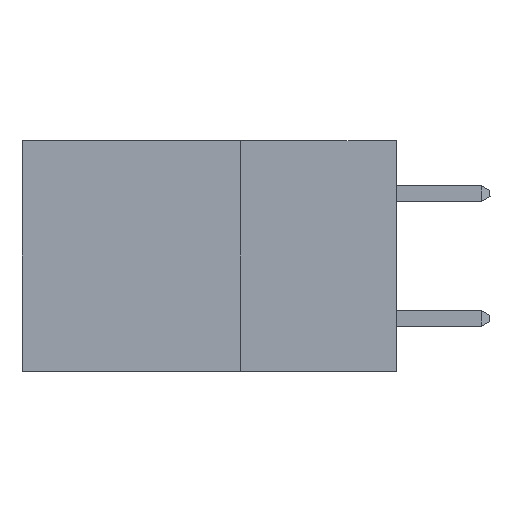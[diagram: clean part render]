
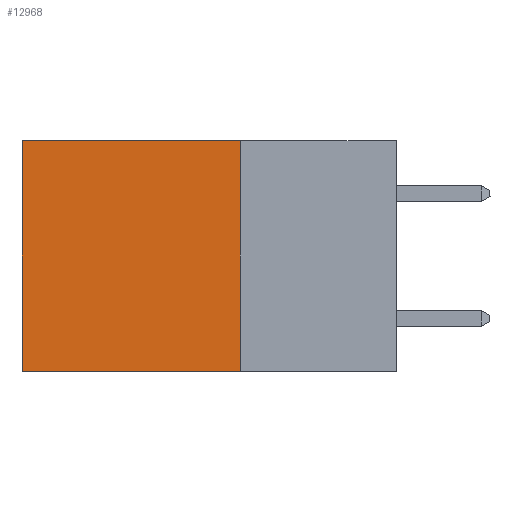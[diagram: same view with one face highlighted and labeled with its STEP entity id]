
A CAD part, left-side view. The second image highlights one B-rep face of the part: STEP entity #12968.
In plain terms, the highlighted planar face has unit normal (-1, 0, 0).
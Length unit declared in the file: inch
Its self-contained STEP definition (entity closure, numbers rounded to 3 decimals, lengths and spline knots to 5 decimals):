
#775 = VECTOR ( 'NONE', #16975, 39.37008 ) ;
#2117 = DIRECTION ( 'NONE',  ( 0., 1., 0. ) ) ;
#3140 = VECTOR ( 'NONE', #21736, 39.37008 ) ;
#4056 = VERTEX_POINT ( 'NONE', #4075 ) ;
#4075 = CARTESIAN_POINT ( 'NONE',  ( 0.298, 0.25, -0.37 ) ) ;
#4980 = LINE ( 'NONE', #5297, #9518 ) ;
#5297 = CARTESIAN_POINT ( 'NONE',  ( 0.298, 0.6, 0. ) ) ;
#9518 = VECTOR ( 'NONE', #20437, 39.37008 ) ;
#9563 = LINE ( 'NONE', #11485, #775 ) ;
#9631 = EDGE_CURVE ( 'NONE', #18186, #13201, #4980, .T. ) ;
#10125 = ORIENTED_EDGE ( 'NONE', *, *, #11398, .T. ) ;
#10546 = LINE ( 'NONE', #20083, #3140 ) ;
#11398 = EDGE_CURVE ( 'NONE', #17300, #18186, #17979, .T. ) ;
#11485 = CARTESIAN_POINT ( 'NONE',  ( 0.298, 0.25, -0.37 ) ) ;
#11583 = CARTESIAN_POINT ( 'NONE',  ( 0.298, 0.25, 0. ) ) ;
#12537 = CARTESIAN_POINT ( 'NONE',  ( 0.298, 0.25, 0. ) ) ;
#12762 = AXIS2_PLACEMENT_3D ( 'NONE', #12537, #23420, #14628 ) ;
#12907 = VECTOR ( 'NONE', #2117, 39.37008 ) ;
#12968 = ADVANCED_FACE ( 'NONE', ( #13417 ), #21691, .F. ) ;
#13201 = VERTEX_POINT ( 'NONE', #22154 ) ;
#13417 = FACE_OUTER_BOUND ( 'NONE', #21770, .T. ) ;
#14628 = DIRECTION ( 'NONE',  ( 0., 0., -1. ) ) ;
#15620 = ORIENTED_EDGE ( 'NONE', *, *, #16050, .F. ) ;
#15751 = ORIENTED_EDGE ( 'NONE', *, *, #9631, .T. ) ;
#16050 = EDGE_CURVE ( 'NONE', #4056, #13201, #9563, .T. ) ;
#16536 = EDGE_CURVE ( 'NONE', #17300, #4056, #10546, .T. ) ;
#16975 = DIRECTION ( 'NONE',  ( 0., 1., 0. ) ) ;
#17300 = VERTEX_POINT ( 'NONE', #11583 ) ;
#17979 = LINE ( 'NONE', #20486, #12907 ) ;
#18186 = VERTEX_POINT ( 'NONE', #22508 ) ;
#20083 = CARTESIAN_POINT ( 'NONE',  ( 0.298, 0.25, 0. ) ) ;
#20437 = DIRECTION ( 'NONE',  ( 0., 0., -1. ) ) ;
#20486 = CARTESIAN_POINT ( 'NONE',  ( 0.298, 0.25, 0. ) ) ;
#21691 = PLANE ( 'NONE',  #12762 ) ;
#21736 = DIRECTION ( 'NONE',  ( 0., 0., -1. ) ) ;
#21770 = EDGE_LOOP ( 'NONE', ( #15751, #15620, #23020, #10125 ) ) ;
#22154 = CARTESIAN_POINT ( 'NONE',  ( 0.298, 0.6, -0.37 ) ) ;
#22508 = CARTESIAN_POINT ( 'NONE',  ( 0.298, 0.6, 0. ) ) ;
#23020 = ORIENTED_EDGE ( 'NONE', *, *, #16536, .F. ) ;
#23420 = DIRECTION ( 'NONE',  ( 1., 0., 0. ) ) ;
